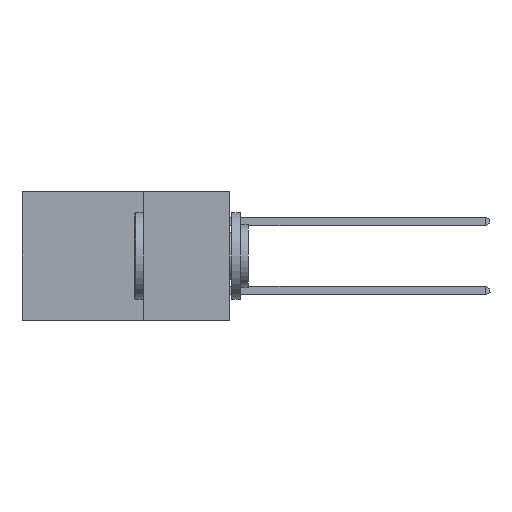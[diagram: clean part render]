
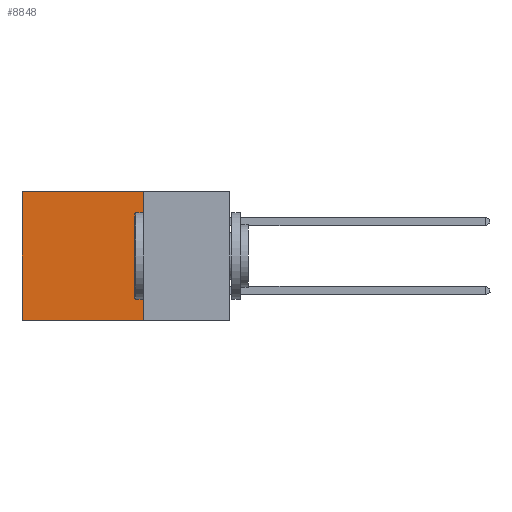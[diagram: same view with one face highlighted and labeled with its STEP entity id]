
A CAD part, left-side view. The second image highlights one B-rep face of the part: STEP entity #8848.
In plain terms, the highlighted planar face has unit normal (-1, 0, 0).
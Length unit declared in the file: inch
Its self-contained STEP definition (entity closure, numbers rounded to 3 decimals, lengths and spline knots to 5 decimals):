
#1687 = CARTESIAN_POINT ( 'NONE',  ( 0.298, 0.25, 0. ) ) ;
#3357 = LINE ( 'NONE', #17450, #18402 ) ;
#3822 = EDGE_CURVE ( 'NONE', #6019, #12971, #3357, .T. ) ;
#5120 = CARTESIAN_POINT ( 'NONE',  ( 0.298, 0.25, -0.37 ) ) ;
#6019 = VERTEX_POINT ( 'NONE', #1687 ) ;
#6106 = VECTOR ( 'NONE', #13570, 39.37008 ) ;
#6256 = CARTESIAN_POINT ( 'NONE',  ( 0.298, 0.25, 0. ) ) ;
#6695 = ORIENTED_EDGE ( 'NONE', *, *, #3822, .T. ) ;
#7078 = PLANE ( 'NONE',  #16240 ) ;
#7264 = DIRECTION ( 'NONE',  ( 0., 1., 0. ) ) ;
#7282 = LINE ( 'NONE', #8633, #10004 ) ;
#7658 = CARTESIAN_POINT ( 'NONE',  ( 0.298, 0.6, 0. ) ) ;
#8246 = EDGE_LOOP ( 'NONE', ( #10152, #16093, #8643, #6695 ) ) ;
#8633 = CARTESIAN_POINT ( 'NONE',  ( 0.298, 0.25, -0.37 ) ) ;
#8643 = ORIENTED_EDGE ( 'NONE', *, *, #12903, .F. ) ;
#8848 = ADVANCED_FACE ( 'NONE', ( #9470 ), #7078, .F. ) ;
#9469 = VECTOR ( 'NONE', #11964, 39.37008 ) ;
#9470 = FACE_OUTER_BOUND ( 'NONE', #8246, .T. ) ;
#10004 = VECTOR ( 'NONE', #14284, 39.37008 ) ;
#10008 = DIRECTION ( 'NONE',  ( 0., 0., -1. ) ) ;
#10128 = CARTESIAN_POINT ( 'NONE',  ( 0.298, 0.6, -0.37 ) ) ;
#10152 = ORIENTED_EDGE ( 'NONE', *, *, #17207, .T. ) ;
#10184 = VERTEX_POINT ( 'NONE', #5120 ) ;
#10600 = LINE ( 'NONE', #14809, #9469 ) ;
#11040 = VERTEX_POINT ( 'NONE', #10128 ) ;
#11964 = DIRECTION ( 'NONE',  ( 0., 0., -1. ) ) ;
#12286 = EDGE_CURVE ( 'NONE', #10184, #11040, #7282, .T. ) ;
#12903 = EDGE_CURVE ( 'NONE', #6019, #10184, #14547, .T. ) ;
#12971 = VERTEX_POINT ( 'NONE', #7658 ) ;
#13570 = DIRECTION ( 'NONE',  ( 0., 0., -1. ) ) ;
#14276 = DIRECTION ( 'NONE',  ( 1., 0., 0. ) ) ;
#14284 = DIRECTION ( 'NONE',  ( 0., 1., 0. ) ) ;
#14547 = LINE ( 'NONE', #6256, #6106 ) ;
#14809 = CARTESIAN_POINT ( 'NONE',  ( 0.298, 0.6, 0. ) ) ;
#15825 = CARTESIAN_POINT ( 'NONE',  ( 0.298, 0.25, 0. ) ) ;
#16093 = ORIENTED_EDGE ( 'NONE', *, *, #12286, .F. ) ;
#16240 = AXIS2_PLACEMENT_3D ( 'NONE', #15825, #14276, #10008 ) ;
#17207 = EDGE_CURVE ( 'NONE', #12971, #11040, #10600, .T. ) ;
#17450 = CARTESIAN_POINT ( 'NONE',  ( 0.298, 0.25, 0. ) ) ;
#18402 = VECTOR ( 'NONE', #7264, 39.37008 ) ;
